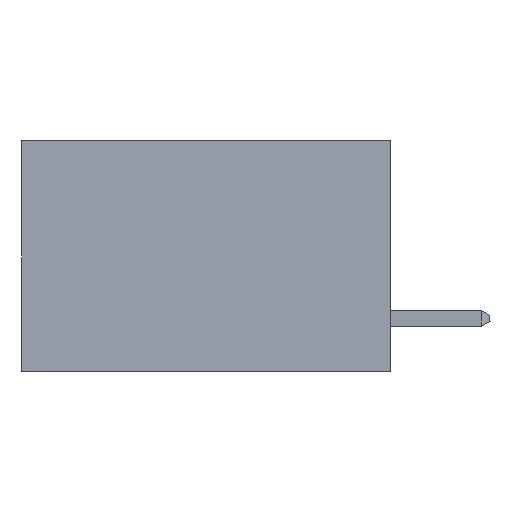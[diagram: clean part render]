
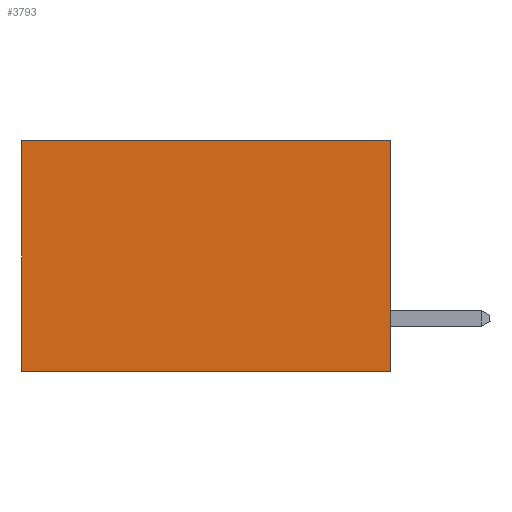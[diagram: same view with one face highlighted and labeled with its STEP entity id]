
A CAD part, left-side view. The second image highlights one B-rep face of the part: STEP entity #3793.
In plain terms, the highlighted planar face has unit normal (-1, 0, 0).
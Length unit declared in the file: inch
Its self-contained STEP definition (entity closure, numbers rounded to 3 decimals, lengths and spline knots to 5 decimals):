
#384 = VECTOR ( 'NONE', #20979, 39.37008 ) ;
#2898 = EDGE_CURVE ( 'NONE', #3599, #8594, #22811, .T. ) ;
#3486 = CARTESIAN_POINT ( 'NONE',  ( 0.277, 0., 0. ) ) ;
#3599 = VERTEX_POINT ( 'NONE', #25625 ) ;
#3793 = ADVANCED_FACE ( 'NONE', ( #21516 ), #16168, .F. ) ;
#4322 = LINE ( 'NONE', #17598, #9896 ) ;
#4970 = DIRECTION ( 'NONE',  ( 0., 1., 0. ) ) ;
#5219 = EDGE_CURVE ( 'NONE', #6860, #19969, #24393, .T. ) ;
#6425 = CARTESIAN_POINT ( 'NONE',  ( 0.277, 0., -0.37 ) ) ;
#6860 = VERTEX_POINT ( 'NONE', #3486 ) ;
#8527 = ORIENTED_EDGE ( 'NONE', *, *, #13797, .F. ) ;
#8594 = VERTEX_POINT ( 'NONE', #26454 ) ;
#8811 = CARTESIAN_POINT ( 'NONE',  ( 0.277, 0., -0.37 ) ) ;
#9896 = VECTOR ( 'NONE', #4970, 39.37008 ) ;
#10134 = VECTOR ( 'NONE', #23289, 39.37008 ) ;
#10289 = ORIENTED_EDGE ( 'NONE', *, *, #27020, .T. ) ;
#10408 = ORIENTED_EDGE ( 'NONE', *, *, #5219, .F. ) ;
#10808 = LINE ( 'NONE', #6425, #10134 ) ;
#13797 = EDGE_CURVE ( 'NONE', #19969, #8594, #10808, .T. ) ;
#15711 = CARTESIAN_POINT ( 'NONE',  ( 0.277, 0., -0.37 ) ) ;
#15784 = DIRECTION ( 'NONE',  ( 0., 0., -1. ) ) ;
#15814 = DIRECTION ( 'NONE',  ( 1., 0., 0. ) ) ;
#16059 = CARTESIAN_POINT ( 'NONE',  ( 0.277, 0., -0.37 ) ) ;
#16168 = PLANE ( 'NONE',  #23025 ) ;
#17176 = DIRECTION ( 'NONE',  ( 0., 0., -1. ) ) ;
#17598 = CARTESIAN_POINT ( 'NONE',  ( 0.277, 0., 0. ) ) ;
#18853 = VECTOR ( 'NONE', #17176, 39.37008 ) ;
#19969 = VERTEX_POINT ( 'NONE', #8811 ) ;
#20979 = DIRECTION ( 'NONE',  ( 0., 0., -1. ) ) ;
#21264 = EDGE_LOOP ( 'NONE', ( #23146, #8527, #10408, #10289 ) ) ;
#21314 = CARTESIAN_POINT ( 'NONE',  ( 0.277, 0.59, -0.37 ) ) ;
#21516 = FACE_OUTER_BOUND ( 'NONE', #21264, .T. ) ;
#22811 = LINE ( 'NONE', #21314, #384 ) ;
#23025 = AXIS2_PLACEMENT_3D ( 'NONE', #16059, #15814, #15784 ) ;
#23146 = ORIENTED_EDGE ( 'NONE', *, *, #2898, .T. ) ;
#23289 = DIRECTION ( 'NONE',  ( 0., 1., 0. ) ) ;
#24393 = LINE ( 'NONE', #15711, #18853 ) ;
#25625 = CARTESIAN_POINT ( 'NONE',  ( 0.277, 0.59, 0. ) ) ;
#26454 = CARTESIAN_POINT ( 'NONE',  ( 0.277, 0.59, -0.37 ) ) ;
#27020 = EDGE_CURVE ( 'NONE', #6860, #3599, #4322, .T. ) ;
